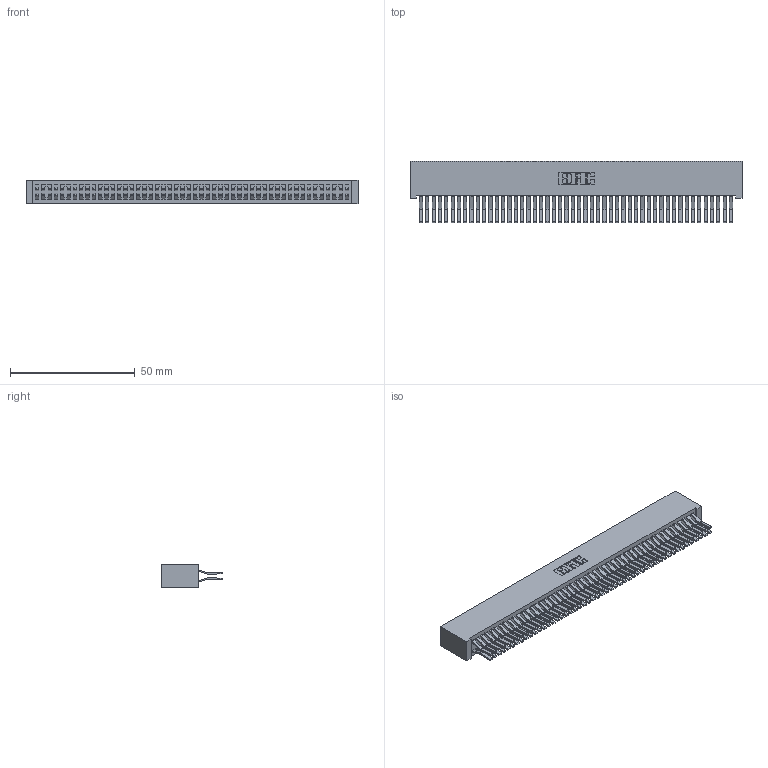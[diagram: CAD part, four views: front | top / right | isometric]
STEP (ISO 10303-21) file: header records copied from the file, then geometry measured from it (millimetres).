
FILE_DESCRIPTION (( 'STEP AP203' ), '1' );
FILE_NAME ('342-100-560-201.STEP', '2018-08-14T04:58:47', ( '' ), ( '' ), 'SwSTEP 2.0', 'SolidWorks 2016', '' );
FILE_SCHEMA (( 'CONFIG_CONTROL_DESIGN' ));
Length unit declared in the file: inch
Products named in the file (3): 342 Part_Lugless; 345-292-001_560 Tail; 342-100-560-201
Assembly tree (101 placements, depth 2):
  342-100-560-201
    342 Part_Lugless
    345-292-001_560 Tail  x100
Bounding box: 133.25 x 24.78 x 9.4 mm (x, y, z)
Volume: 13106.3 mm3; surface area: 23551.3 mm2
Topology: 101 solids, 101 shells, 5502 faces, 16375 edges, 10782 vertices
Faces by surface type: plane 3662, cylinder 1840
Entity records: 30811 total; most frequent: CARTESIAN_POINT 5094, ORIENTED_EDGE 5030, DIRECTION 4335, EDGE_CURVE 2515, VECTOR 2391, LINE 2391, VERTEX_POINT 1674, AXIS2_PLACEMENT_3D 972
